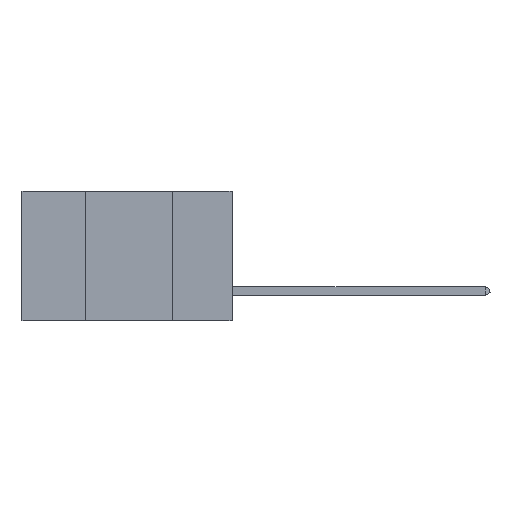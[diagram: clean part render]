
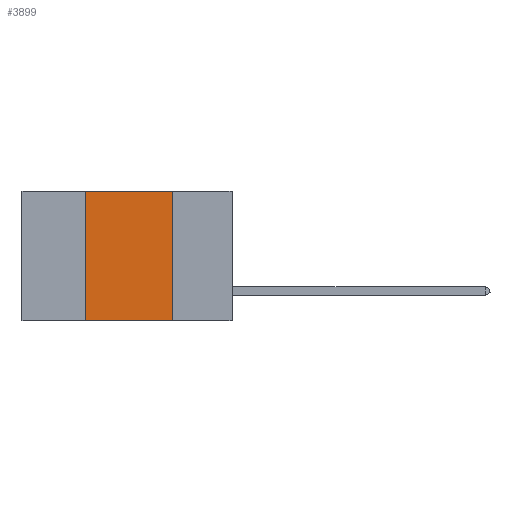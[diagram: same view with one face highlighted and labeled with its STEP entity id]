
A CAD part, left-side view. The second image highlights one B-rep face of the part: STEP entity #3899.
In plain terms, the highlighted planar face has unit normal (-1, 0, 0).
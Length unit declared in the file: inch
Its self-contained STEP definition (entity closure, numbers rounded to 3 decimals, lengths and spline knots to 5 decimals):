
#101 = LINE ( 'NONE', #10395, #9738 ) ;
#245 = VERTEX_POINT ( 'NONE', #1765 ) ;
#439 = EDGE_CURVE ( 'NONE', #8010, #5260, #6867, .T. ) ;
#524 = PLANE ( 'NONE',  #4072 ) ;
#602 = DIRECTION ( 'NONE',  ( 0., 0., -1. ) ) ;
#712 = DIRECTION ( 'NONE',  ( 0., 0., -1. ) ) ;
#816 = ORIENTED_EDGE ( 'NONE', *, *, #6190, .T. ) ;
#1203 = VECTOR ( 'NONE', #2117, 39.37008 ) ;
#1765 = CARTESIAN_POINT ( 'NONE',  ( 0., 0.42, -0.37 ) ) ;
#1805 = CARTESIAN_POINT ( 'NONE',  ( 0., 0.17, -0.37 ) ) ;
#1807 = DIRECTION ( 'NONE',  ( 0., -1., 0. ) ) ;
#2117 = DIRECTION ( 'NONE',  ( 0., -1., 0. ) ) ;
#2849 = DIRECTION ( 'NONE',  ( 0., 0., 1. ) ) ;
#3343 = EDGE_CURVE ( 'NONE', #5260, #10966, #10097, .T. ) ;
#3899 = ADVANCED_FACE ( 'NONE', ( #7221 ), #524, .F. ) ;
#4014 = CARTESIAN_POINT ( 'NONE',  ( 0., 0.6, 0. ) ) ;
#4060 = CARTESIAN_POINT ( 'NONE',  ( 0., 0.17, 0. ) ) ;
#4072 = AXIS2_PLACEMENT_3D ( 'NONE', #4014, #6491, #602 ) ;
#4699 = CARTESIAN_POINT ( 'NONE',  ( 0., 0.6, 0. ) ) ;
#4891 = LINE ( 'NONE', #8814, #5563 ) ;
#5260 = VERTEX_POINT ( 'NONE', #4060 ) ;
#5431 = ORIENTED_EDGE ( 'NONE', *, *, #3343, .F. ) ;
#5563 = VECTOR ( 'NONE', #2849, 39.37008 ) ;
#5612 = EDGE_LOOP ( 'NONE', ( #5431, #10256, #6674, #816 ) ) ;
#5983 = EDGE_CURVE ( 'NONE', #245, #8010, #4891, .T. ) ;
#6190 = EDGE_CURVE ( 'NONE', #245, #10966, #101, .T. ) ;
#6281 = VECTOR ( 'NONE', #712, 39.37008 ) ;
#6491 = DIRECTION ( 'NONE',  ( 1., 0., 0. ) ) ;
#6654 = CARTESIAN_POINT ( 'NONE',  ( 0., 0.17, 0. ) ) ;
#6674 = ORIENTED_EDGE ( 'NONE', *, *, #5983, .F. ) ;
#6867 = LINE ( 'NONE', #4699, #1203 ) ;
#7221 = FACE_OUTER_BOUND ( 'NONE', #5612, .T. ) ;
#8010 = VERTEX_POINT ( 'NONE', #8383 ) ;
#8383 = CARTESIAN_POINT ( 'NONE',  ( 0., 0.42, 0. ) ) ;
#8814 = CARTESIAN_POINT ( 'NONE',  ( 0., 0.42, 0. ) ) ;
#9738 = VECTOR ( 'NONE', #1807, 39.37008 ) ;
#10097 = LINE ( 'NONE', #6654, #6281 ) ;
#10256 = ORIENTED_EDGE ( 'NONE', *, *, #439, .F. ) ;
#10395 = CARTESIAN_POINT ( 'NONE',  ( 0., 0.6, -0.37 ) ) ;
#10966 = VERTEX_POINT ( 'NONE', #1805 ) ;
